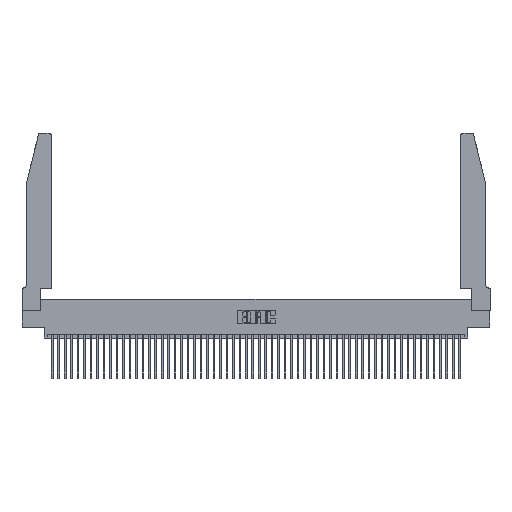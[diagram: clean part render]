
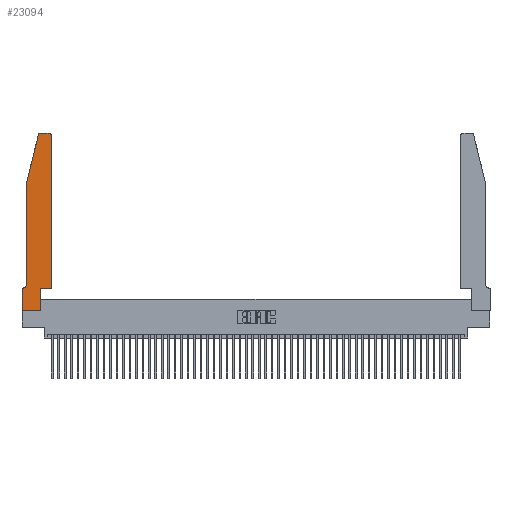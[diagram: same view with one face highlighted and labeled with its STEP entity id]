
A CAD part, top view. The second image highlights one B-rep face of the part: STEP entity #23094.
In plain terms, the highlighted planar face has unit normal (0, 0, 1).
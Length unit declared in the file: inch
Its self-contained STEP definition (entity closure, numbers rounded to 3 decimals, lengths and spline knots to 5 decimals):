
#483 = EDGE_LOOP ( 'NONE', ( #51722, #12782, #34180, #13265, #25897, #18951, #40319, #45356, #38459, #18346, #32820, #1896 ) ) ;
#573 = DIRECTION ( 'NONE',  ( 0., 0., 1. ) ) ;
#862 = DIRECTION ( 'NONE',  ( 1., 0., 0. ) ) ;
#1478 = DIRECTION ( 'NONE',  ( 0., 1., 0. ) ) ;
#1706 = AXIS2_PLACEMENT_3D ( 'NONE', #24823, #573, #28841 ) ;
#1896 = ORIENTED_EDGE ( 'NONE', *, *, #48644, .T. ) ;
#3951 = VECTOR ( 'NONE', #43624, 39.37008 ) ;
#3988 = VERTEX_POINT ( 'NONE', #32416 ) ;
#4868 = LINE ( 'NONE', #38974, #35767 ) ;
#5760 = VERTEX_POINT ( 'NONE', #9703 ) ;
#7336 = VECTOR ( 'NONE', #15465, 39.37008 ) ;
#8039 = VERTEX_POINT ( 'NONE', #48012 ) ;
#8309 = EDGE_CURVE ( 'NONE', #22291, #35835, #45286, .T. ) ;
#8822 = VERTEX_POINT ( 'NONE', #48639 ) ;
#8962 = CARTESIAN_POINT ( 'NONE',  ( 0.2605, 2.75, 0.37 ) ) ;
#9010 = AXIS2_PLACEMENT_3D ( 'NONE', #27458, #51660, #27633 ) ;
#9703 = CARTESIAN_POINT ( 'NONE',  ( 0.284, 2.75, 0.37 ) ) ;
#10059 = LINE ( 'NONE', #19369, #51532 ) ;
#10541 = CARTESIAN_POINT ( 'NONE',  ( 0., 0., 0.37 ) ) ;
#11422 = CARTESIAN_POINT ( 'NONE',  ( 0., 0., 0.37 ) ) ;
#11895 = EDGE_CURVE ( 'NONE', #37873, #41956, #31499, .T. ) ;
#12556 = CARTESIAN_POINT ( 'NONE',  ( 0.0755, 2., 0.37 ) ) ;
#12782 = ORIENTED_EDGE ( 'NONE', *, *, #47892, .T. ) ;
#13042 = DIRECTION ( 'NONE',  ( -1., 0., 0. ) ) ;
#13265 = ORIENTED_EDGE ( 'NONE', *, *, #32199, .T. ) ;
#13487 = LINE ( 'NONE', #39595, #3951 ) ;
#13488 = CARTESIAN_POINT ( 'NONE',  ( 0.2865, 0., 0.37 ) ) ;
#15465 = DIRECTION ( 'NONE',  ( 1., 0., 0. ) ) ;
#15888 = CARTESIAN_POINT ( 'NONE',  ( 0.4505, 0.35, 0.37 ) ) ;
#16334 = EDGE_CURVE ( 'NONE', #45101, #24099, #39477, .T. ) ;
#17223 = VECTOR ( 'NONE', #13042, 39.37008 ) ;
#17640 = DIRECTION ( 'NONE',  ( 0., 0., -1. ) ) ;
#18346 = ORIENTED_EDGE ( 'NONE', *, *, #50803, .T. ) ;
#18951 = ORIENTED_EDGE ( 'NONE', *, *, #48303, .T. ) ;
#19369 = CARTESIAN_POINT ( 'NONE',  ( 0.2865, 0.35, 0.37 ) ) ;
#19491 = EDGE_CURVE ( 'NONE', #8039, #31208, #29174, .T. ) ;
#19495 = EDGE_CURVE ( 'NONE', #35276, #5760, #49234, .T. ) ;
#20655 = CIRCLE ( 'NONE', #51961, 0.03 ) ;
#21412 = VECTOR ( 'NONE', #28085, 39.37008 ) ;
#22291 = VERTEX_POINT ( 'NONE', #44787 ) ;
#22449 = AXIS2_PLACEMENT_3D ( 'NONE', #41689, #17640, #45740 ) ;
#22637 = CIRCLE ( 'NONE', #1706, 0.03 ) ;
#22724 = DIRECTION ( 'NONE',  ( 0., -1., 0. ) ) ;
#23094 = ADVANCED_FACE ( 'NONE', ( #36590 ), #23604, .T. ) ;
#23413 = DIRECTION ( 'NONE',  ( 0., 1., 0. ) ) ;
#23604 = PLANE ( 'NONE',  #9010 ) ;
#23872 = CARTESIAN_POINT ( 'NONE',  ( 0.0755, 2., 0.37 ) ) ;
#24099 = VERTEX_POINT ( 'NONE', #13488 ) ;
#24823 = CARTESIAN_POINT ( 'NONE',  ( 0.284, 2.72, 0.37 ) ) ;
#25114 = DIRECTION ( 'NONE',  ( 0., 0., 1. ) ) ;
#25897 = ORIENTED_EDGE ( 'NONE', *, *, #8309, .T. ) ;
#26775 = LINE ( 'NONE', #10541, #37469 ) ;
#27458 = CARTESIAN_POINT ( 'NONE',  ( 0., 0.35, 0.37 ) ) ;
#27633 = DIRECTION ( 'NONE',  ( 1., 0., 0. ) ) ;
#28085 = DIRECTION ( 'NONE',  ( 0., -1., 0. ) ) ;
#28841 = DIRECTION ( 'NONE',  ( 1., 0., 0. ) ) ;
#29042 = CARTESIAN_POINT ( 'NONE',  ( 0.0755, 2., 0.37 ) ) ;
#29174 = LINE ( 'NONE', #29042, #38584 ) ;
#31208 = VERTEX_POINT ( 'NONE', #12556 ) ;
#31499 = LINE ( 'NONE', #41648, #51568 ) ;
#32199 = EDGE_CURVE ( 'NONE', #31208, #22291, #41486, .T. ) ;
#32416 = CARTESIAN_POINT ( 'NONE',  ( 0., 0.35, 0.37 ) ) ;
#32820 = ORIENTED_EDGE ( 'NONE', *, *, #11895, .T. ) ;
#33071 = DIRECTION ( 'NONE',  ( -0.239, -0.971, 0. ) ) ;
#34180 = ORIENTED_EDGE ( 'NONE', *, *, #19491, .T. ) ;
#34573 = EDGE_CURVE ( 'NONE', #3988, #45101, #26775, .T. ) ;
#35276 = VERTEX_POINT ( 'NONE', #35639 ) ;
#35639 = CARTESIAN_POINT ( 'NONE',  ( 0.4205, 2.75, 0.37 ) ) ;
#35767 = VECTOR ( 'NONE', #43000, 39.37008 ) ;
#35835 = VERTEX_POINT ( 'NONE', #38735 ) ;
#36590 = FACE_OUTER_BOUND ( 'NONE', #483, .T. ) ;
#37173 = CARTESIAN_POINT ( 'NONE',  ( 0., 0., 0.37 ) ) ;
#37469 = VECTOR ( 'NONE', #22724, 39.37008 ) ;
#37873 = VERTEX_POINT ( 'NONE', #15888 ) ;
#38368 = EDGE_CURVE ( 'NONE', #24099, #8822, #10059, .T. ) ;
#38459 = ORIENTED_EDGE ( 'NONE', *, *, #38368, .T. ) ;
#38584 = VECTOR ( 'NONE', #33071, 39.37008 ) ;
#38735 = CARTESIAN_POINT ( 'NONE',  ( 0.0055, 0.35, 0.37 ) ) ;
#38974 = CARTESIAN_POINT ( 'NONE',  ( 0.0755, 0.35, 0.37 ) ) ;
#39477 = LINE ( 'NONE', #11422, #7336 ) ;
#39595 = CARTESIAN_POINT ( 'NONE',  ( 0.4505, 0.35, 0.37 ) ) ;
#40319 = ORIENTED_EDGE ( 'NONE', *, *, #34573, .T. ) ;
#41486 = LINE ( 'NONE', #23872, #21412 ) ;
#41648 = CARTESIAN_POINT ( 'NONE',  ( 0.4505, 0.35, 0.37 ) ) ;
#41689 = CARTESIAN_POINT ( 'NONE',  ( 0.0055, 0.42, 0.37 ) ) ;
#41956 = VERTEX_POINT ( 'NONE', #46310 ) ;
#43000 = DIRECTION ( 'NONE',  ( -1., 0., 0. ) ) ;
#43624 = DIRECTION ( 'NONE',  ( 1., 0., 0. ) ) ;
#44787 = CARTESIAN_POINT ( 'NONE',  ( 0.0755, 0.42, 0.37 ) ) ;
#45101 = VERTEX_POINT ( 'NONE', #37173 ) ;
#45286 = CIRCLE ( 'NONE', #22449, 0.07 ) ;
#45356 = ORIENTED_EDGE ( 'NONE', *, *, #16334, .T. ) ;
#45740 = DIRECTION ( 'NONE',  ( -1., 0., 0. ) ) ;
#46310 = CARTESIAN_POINT ( 'NONE',  ( 0.4505, 2.72, 0.37 ) ) ;
#47892 = EDGE_CURVE ( 'NONE', #5760, #8039, #22637, .T. ) ;
#48012 = CARTESIAN_POINT ( 'NONE',  ( 0.25487, 2.72718, 0.37 ) ) ;
#48303 = EDGE_CURVE ( 'NONE', #35835, #3988, #4868, .T. ) ;
#48639 = CARTESIAN_POINT ( 'NONE',  ( 0.2865, 0.35, 0.37 ) ) ;
#48644 = EDGE_CURVE ( 'NONE', #41956, #35276, #20655, .T. ) ;
#49102 = CARTESIAN_POINT ( 'NONE',  ( 0.4205, 2.72, 0.37 ) ) ;
#49234 = LINE ( 'NONE', #8962, #17223 ) ;
#50803 = EDGE_CURVE ( 'NONE', #8822, #37873, #13487, .T. ) ;
#51532 = VECTOR ( 'NONE', #23413, 39.37008 ) ;
#51568 = VECTOR ( 'NONE', #1478, 39.37008 ) ;
#51660 = DIRECTION ( 'NONE',  ( 0., 0., 1. ) ) ;
#51722 = ORIENTED_EDGE ( 'NONE', *, *, #19495, .T. ) ;
#51961 = AXIS2_PLACEMENT_3D ( 'NONE', #49102, #25114, #862 ) ;
